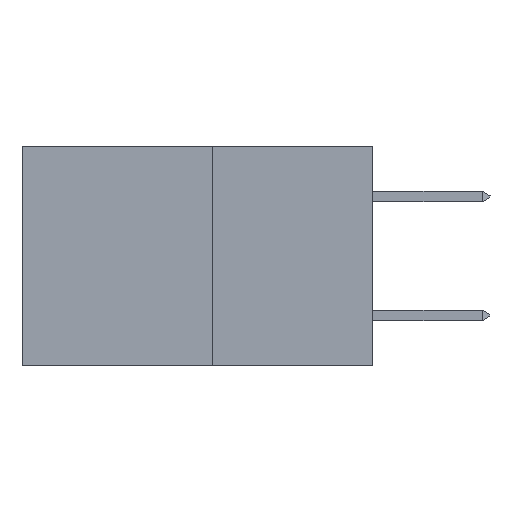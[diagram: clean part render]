
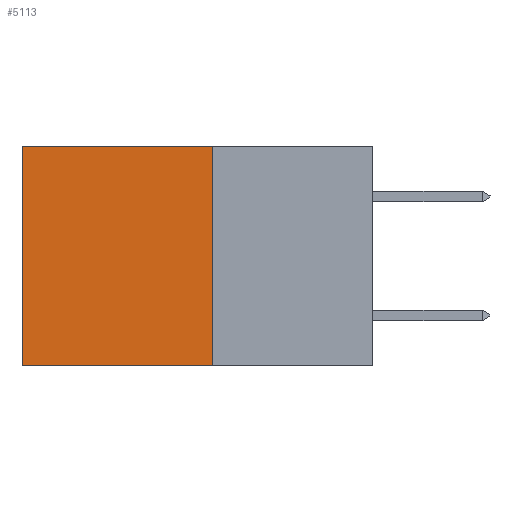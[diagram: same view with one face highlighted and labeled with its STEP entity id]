
A CAD part, left-side view. The second image highlights one B-rep face of the part: STEP entity #5113.
In plain terms, the highlighted planar face has unit normal (-1, 0, 0).
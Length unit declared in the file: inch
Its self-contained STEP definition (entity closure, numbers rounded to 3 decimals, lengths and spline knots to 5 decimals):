
#884 = EDGE_CURVE ( 'NONE', #12039, #26427, #22942, .T. ) ;
#1865 = DIRECTION ( 'NONE',  ( 0., 1., 0. ) ) ;
#2100 = VERTEX_POINT ( 'NONE', #16078 ) ;
#2603 = ORIENTED_EDGE ( 'NONE', *, *, #884, .T. ) ;
#3704 = CARTESIAN_POINT ( 'NONE',  ( 0.277, 0.59, -0.37 ) ) ;
#4113 = VECTOR ( 'NONE', #10803, 39.37008 ) ;
#5113 = ADVANCED_FACE ( 'NONE', ( #16477 ), #14955, .F. ) ;
#5950 = EDGE_CURVE ( 'NONE', #26427, #25215, #21994, .T. ) ;
#7044 = ORIENTED_EDGE ( 'NONE', *, *, #28503, .F. ) ;
#7889 = LINE ( 'NONE', #25276, #20298 ) ;
#9535 = VECTOR ( 'NONE', #1865, 39.37008 ) ;
#10239 = CARTESIAN_POINT ( 'NONE',  ( 0.277, 0.27, -0.37 ) ) ;
#10803 = DIRECTION ( 'NONE',  ( 0., 0., -1. ) ) ;
#11009 = ORIENTED_EDGE ( 'NONE', *, *, #5950, .T. ) ;
#12039 = VERTEX_POINT ( 'NONE', #17189 ) ;
#13051 = CARTESIAN_POINT ( 'NONE',  ( 0.277, 0.59, 0. ) ) ;
#13464 = CARTESIAN_POINT ( 'NONE',  ( 0.277, 0.27, -0.37 ) ) ;
#13508 = DIRECTION ( 'NONE',  ( 0., 0., -1. ) ) ;
#13927 = EDGE_CURVE ( 'NONE', #12039, #2100, #7889, .T. ) ;
#14560 = ORIENTED_EDGE ( 'NONE', *, *, #13927, .F. ) ;
#14955 = PLANE ( 'NONE',  #19178 ) ;
#15981 = VECTOR ( 'NONE', #16829, 39.37008 ) ;
#16078 = CARTESIAN_POINT ( 'NONE',  ( 0.277, 0.27, -0.37 ) ) ;
#16477 = FACE_OUTER_BOUND ( 'NONE', #16737, .T. ) ;
#16737 = EDGE_LOOP ( 'NONE', ( #11009, #7044, #14560, #2603 ) ) ;
#16829 = DIRECTION ( 'NONE',  ( 0., 1., 0. ) ) ;
#16892 = CARTESIAN_POINT ( 'NONE',  ( 0.277, 0.27, 0. ) ) ;
#17189 = CARTESIAN_POINT ( 'NONE',  ( 0.277, 0.27, 0. ) ) ;
#18208 = DIRECTION ( 'NONE',  ( 0., 0., -1. ) ) ;
#19178 = AXIS2_PLACEMENT_3D ( 'NONE', #10239, #27039, #18208 ) ;
#20298 = VECTOR ( 'NONE', #13508, 39.37008 ) ;
#21973 = LINE ( 'NONE', #13464, #9535 ) ;
#21994 = LINE ( 'NONE', #3704, #4113 ) ;
#22942 = LINE ( 'NONE', #16892, #15981 ) ;
#25011 = CARTESIAN_POINT ( 'NONE',  ( 0.277, 0.59, -0.37 ) ) ;
#25215 = VERTEX_POINT ( 'NONE', #25011 ) ;
#25276 = CARTESIAN_POINT ( 'NONE',  ( 0.277, 0.27, -0.37 ) ) ;
#26427 = VERTEX_POINT ( 'NONE', #13051 ) ;
#27039 = DIRECTION ( 'NONE',  ( 1., 0., 0. ) ) ;
#28503 = EDGE_CURVE ( 'NONE', #2100, #25215, #21973, .T. ) ;
